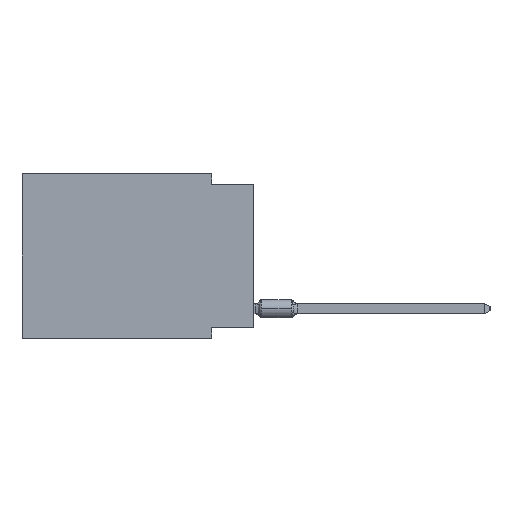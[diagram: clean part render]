
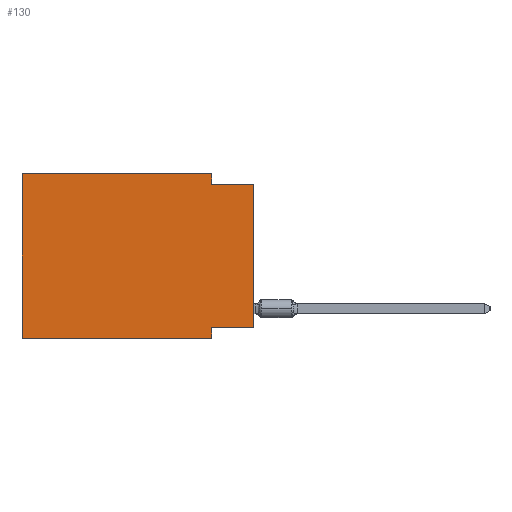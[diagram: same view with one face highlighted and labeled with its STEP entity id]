
A CAD part, left-side view. The second image highlights one B-rep face of the part: STEP entity #130.
In plain terms, the highlighted planar face has unit normal (-1, 0, 0).
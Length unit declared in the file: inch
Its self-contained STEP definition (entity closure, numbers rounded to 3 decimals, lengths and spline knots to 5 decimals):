
#130 = ADVANCED_FACE ( 'NONE', ( #29115 ), #1833, .F. ) ;
#1632 = VECTOR ( 'NONE', #49076, 39.37008 ) ;
#1788 = CARTESIAN_POINT ( 'NONE',  ( 0., 0.55, -0.39 ) ) ;
#1833 = PLANE ( 'NONE',  #18296 ) ;
#2076 = CARTESIAN_POINT ( 'NONE',  ( 0., 0.1, 0. ) ) ;
#3828 = LINE ( 'NONE', #48857, #47445 ) ;
#4298 = CARTESIAN_POINT ( 'NONE',  ( 0., 0.55, 0. ) ) ;
#4444 = EDGE_CURVE ( 'NONE', #41889, #5352, #25685, .T. ) ;
#4696 = VECTOR ( 'NONE', #53728, 39.37008 ) ;
#5352 = VERTEX_POINT ( 'NONE', #42226 ) ;
#6428 = CARTESIAN_POINT ( 'NONE',  ( 0., 0., 0. ) ) ;
#7808 = CARTESIAN_POINT ( 'NONE',  ( 0., 0.1, -0.025 ) ) ;
#8383 = ORIENTED_EDGE ( 'NONE', *, *, #38576, .F. ) ;
#11024 = DIRECTION ( 'NONE',  ( 0., 1., 0. ) ) ;
#11508 = DIRECTION ( 'NONE',  ( 0., 0., 1. ) ) ;
#12032 = CARTESIAN_POINT ( 'NONE',  ( 0., 0., -0.025 ) ) ;
#14462 = VECTOR ( 'NONE', #11024, 39.37008 ) ;
#15351 = DIRECTION ( 'NONE',  ( 0., 0., -1. ) ) ;
#16430 = CARTESIAN_POINT ( 'NONE',  ( 0., 0.1, -0.39 ) ) ;
#16801 = EDGE_CURVE ( 'NONE', #55933, #53627, #3828, .T. ) ;
#17121 = EDGE_CURVE ( 'NONE', #41889, #42084, #39090, .T. ) ;
#18296 = AXIS2_PLACEMENT_3D ( 'NONE', #43531, #20121, #24901 ) ;
#19001 = EDGE_LOOP ( 'NONE', ( #33510, #43188, #46909, #8383, #42006, #50130, #38815, #52091 ) ) ;
#19628 = CARTESIAN_POINT ( 'NONE',  ( 0., 0.1, 0. ) ) ;
#19860 = LINE ( 'NONE', #21015, #32183 ) ;
#20121 = DIRECTION ( 'NONE',  ( 1., 0., 0. ) ) ;
#21015 = CARTESIAN_POINT ( 'NONE',  ( 0., 0.1, -0.39 ) ) ;
#21815 = DIRECTION ( 'NONE',  ( 0., 0., 1. ) ) ;
#24803 = CARTESIAN_POINT ( 'NONE',  ( 0., 0., -0.365 ) ) ;
#24901 = DIRECTION ( 'NONE',  ( 0., 0., -1. ) ) ;
#25685 = LINE ( 'NONE', #24803, #14462 ) ;
#29115 = FACE_OUTER_BOUND ( 'NONE', #19001, .T. ) ;
#30320 = LINE ( 'NONE', #12032, #4696 ) ;
#31197 = VECTOR ( 'NONE', #11508, 39.37008 ) ;
#32183 = VECTOR ( 'NONE', #15351, 39.37008 ) ;
#33510 = ORIENTED_EDGE ( 'NONE', *, *, #17121, .T. ) ;
#34159 = LINE ( 'NONE', #1788, #1632 ) ;
#37049 = DIRECTION ( 'NONE',  ( 0., 0., -1. ) ) ;
#37343 = LINE ( 'NONE', #19628, #43691 ) ;
#38576 = EDGE_CURVE ( 'NONE', #53627, #42489, #52238, .T. ) ;
#38815 = ORIENTED_EDGE ( 'NONE', *, *, #59039, .F. ) ;
#39090 = LINE ( 'NONE', #6428, #31197 ) ;
#39162 = VERTEX_POINT ( 'NONE', #16430 ) ;
#40951 = CARTESIAN_POINT ( 'NONE',  ( 0., 0.55, -0.39 ) ) ;
#41544 = CARTESIAN_POINT ( 'NONE',  ( 0., 0., -0.025 ) ) ;
#41625 = VECTOR ( 'NONE', #42636, 39.37008 ) ;
#41889 = VERTEX_POINT ( 'NONE', #44569 ) ;
#42006 = ORIENTED_EDGE ( 'NONE', *, *, #16801, .F. ) ;
#42084 = VERTEX_POINT ( 'NONE', #41544 ) ;
#42226 = CARTESIAN_POINT ( 'NONE',  ( 0., 0.1, -0.365 ) ) ;
#42489 = VERTEX_POINT ( 'NONE', #2076 ) ;
#42636 = DIRECTION ( 'NONE',  ( 0., -1., 0. ) ) ;
#43188 = ORIENTED_EDGE ( 'NONE', *, *, #43999, .F. ) ;
#43531 = CARTESIAN_POINT ( 'NONE',  ( 0., 0.55, 0. ) ) ;
#43691 = VECTOR ( 'NONE', #37049, 39.37008 ) ;
#43999 = EDGE_CURVE ( 'NONE', #49668, #42084, #30320, .T. ) ;
#44569 = CARTESIAN_POINT ( 'NONE',  ( 0., 0., -0.365 ) ) ;
#46909 = ORIENTED_EDGE ( 'NONE', *, *, #57321, .F. ) ;
#47445 = VECTOR ( 'NONE', #21815, 39.37008 ) ;
#48857 = CARTESIAN_POINT ( 'NONE',  ( 0., 0.55, 0. ) ) ;
#49076 = DIRECTION ( 'NONE',  ( 0., -1., 0. ) ) ;
#49668 = VERTEX_POINT ( 'NONE', #7808 ) ;
#50130 = ORIENTED_EDGE ( 'NONE', *, *, #58267, .T. ) ;
#52091 = ORIENTED_EDGE ( 'NONE', *, *, #4444, .F. ) ;
#52238 = LINE ( 'NONE', #57042, #41625 ) ;
#53627 = VERTEX_POINT ( 'NONE', #4298 ) ;
#53728 = DIRECTION ( 'NONE',  ( 0., -1., 0. ) ) ;
#55933 = VERTEX_POINT ( 'NONE', #40951 ) ;
#57042 = CARTESIAN_POINT ( 'NONE',  ( 0., 0.55, 0. ) ) ;
#57321 = EDGE_CURVE ( 'NONE', #42489, #49668, #37343, .T. ) ;
#58267 = EDGE_CURVE ( 'NONE', #55933, #39162, #34159, .T. ) ;
#59039 = EDGE_CURVE ( 'NONE', #5352, #39162, #19860, .T. ) ;
